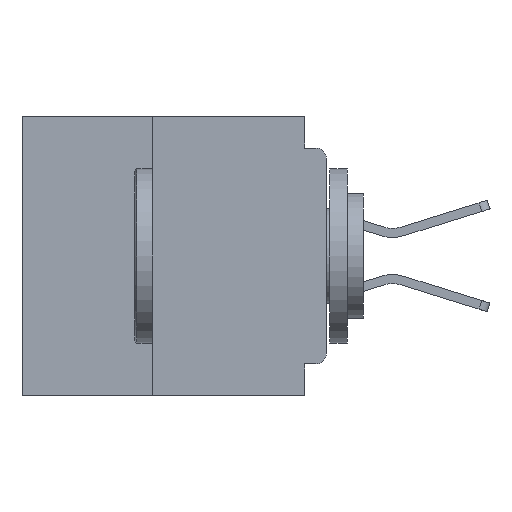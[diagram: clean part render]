
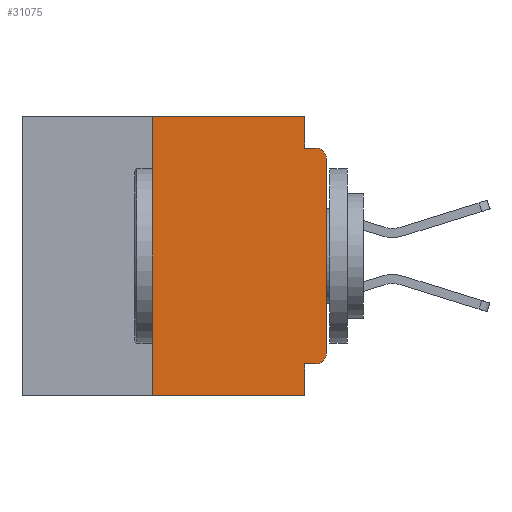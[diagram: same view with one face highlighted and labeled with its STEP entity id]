
A CAD part, left-side view. The second image highlights one B-rep face of the part: STEP entity #31075.
In plain terms, the highlighted planar face has unit normal (-1, 0, 0).
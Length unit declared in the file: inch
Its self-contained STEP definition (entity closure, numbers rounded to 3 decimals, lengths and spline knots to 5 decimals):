
#93 = CARTESIAN_POINT ( 'NONE',  ( 0., 0.015, -0.06 ) ) ;
#220 = EDGE_CURVE ( 'NONE', #1124, #21345, #11025, .T. ) ;
#912 = VERTEX_POINT ( 'NONE', #42246 ) ;
#926 = VECTOR ( 'NONE', #17626, 39.37008 ) ;
#1124 = VERTEX_POINT ( 'NONE', #22435 ) ;
#1366 = AXIS2_PLACEMENT_3D ( 'NONE', #93, #27262, #4027 ) ;
#1625 = DIRECTION ( 'NONE',  ( 0., -1., 0. ) ) ;
#2060 = ORIENTED_EDGE ( 'NONE', *, *, #20416, .F. ) ;
#3222 = CARTESIAN_POINT ( 'NONE',  ( 0., 0., -0.34 ) ) ;
#3652 = LINE ( 'NONE', #19843, #23049 ) ;
#3654 = CARTESIAN_POINT ( 'NONE',  ( 0., 0., -0.045 ) ) ;
#4017 = DIRECTION ( 'NONE',  ( 0., 0., -1. ) ) ;
#4027 = DIRECTION ( 'NONE',  ( 0., 0., -1. ) ) ;
#4839 = EDGE_CURVE ( 'NONE', #48604, #32258, #38915, .T. ) ;
#5879 = CARTESIAN_POINT ( 'NONE',  ( 0., 0.031, -0.4 ) ) ;
#5947 = CARTESIAN_POINT ( 'NONE',  ( 0., 0., -0.355 ) ) ;
#6257 = CIRCLE ( 'NONE', #8171, 0.015 ) ;
#6367 = VECTOR ( 'NONE', #1625, 39.37008 ) ;
#6814 = DIRECTION ( 'NONE',  ( 0., 0., -1. ) ) ;
#7011 = CARTESIAN_POINT ( 'NONE',  ( 0., 0.031, -0.045 ) ) ;
#7344 = EDGE_CURVE ( 'NONE', #23787, #32258, #38089, .T. ) ;
#7487 = AXIS2_PLACEMENT_3D ( 'NONE', #23342, #27258, #4017 ) ;
#8171 = AXIS2_PLACEMENT_3D ( 'NONE', #22009, #48765, #25930 ) ;
#8413 = ORIENTED_EDGE ( 'NONE', *, *, #29179, .T. ) ;
#8745 = CARTESIAN_POINT ( 'NONE',  ( 0., 0.015, -0.355 ) ) ;
#9720 = DIRECTION ( 'NONE',  ( 0., 0., 1. ) ) ;
#9764 = EDGE_CURVE ( 'NONE', #22060, #38439, #40261, .T. ) ;
#9874 = DIRECTION ( 'NONE',  ( 0., 1., 0. ) ) ;
#10141 = EDGE_CURVE ( 'NONE', #17480, #48604, #3652, .T. ) ;
#10224 = VERTEX_POINT ( 'NONE', #20346 ) ;
#11025 = LINE ( 'NONE', #42418, #12229 ) ;
#11294 = LINE ( 'NONE', #5879, #926 ) ;
#11727 = ORIENTED_EDGE ( 'NONE', *, *, #33184, .F. ) ;
#11747 = CARTESIAN_POINT ( 'NONE',  ( 0., 0.015, -0.045 ) ) ;
#12229 = VECTOR ( 'NONE', #9720, 39.37008 ) ;
#12519 = CARTESIAN_POINT ( 'NONE',  ( 0., 0.25, 0. ) ) ;
#13528 = VECTOR ( 'NONE', #6814, 39.37008 ) ;
#14479 = CARTESIAN_POINT ( 'NONE',  ( 0., 0.437, -0.4 ) ) ;
#17480 = VERTEX_POINT ( 'NONE', #3222 ) ;
#17592 = VECTOR ( 'NONE', #19287, 39.37008 ) ;
#17626 = DIRECTION ( 'NONE',  ( 0., 0., -1. ) ) ;
#18021 = ORIENTED_EDGE ( 'NONE', *, *, #9764, .F. ) ;
#18552 = ORIENTED_EDGE ( 'NONE', *, *, #23056, .F. ) ;
#19287 = DIRECTION ( 'NONE',  ( 0., -1., 0. ) ) ;
#19843 = CARTESIAN_POINT ( 'NONE',  ( 0., 0., 0. ) ) ;
#20346 = CARTESIAN_POINT ( 'NONE',  ( 0., 0.031, -0.4 ) ) ;
#20416 = EDGE_CURVE ( 'NONE', #912, #23787, #23808, .T. ) ;
#21345 = VERTEX_POINT ( 'NONE', #12519 ) ;
#22009 = CARTESIAN_POINT ( 'NONE',  ( 0., 0.015, -0.34 ) ) ;
#22060 = VERTEX_POINT ( 'NONE', #8745 ) ;
#22105 = ORIENTED_EDGE ( 'NONE', *, *, #30466, .T. ) ;
#22252 = CARTESIAN_POINT ( 'NONE',  ( 0., 0.031, 0. ) ) ;
#22435 = CARTESIAN_POINT ( 'NONE',  ( 0., 0.25, -0.4 ) ) ;
#23049 = VECTOR ( 'NONE', #23716, 39.37008 ) ;
#23056 = EDGE_CURVE ( 'NONE', #38439, #10224, #11294, .T. ) ;
#23342 = CARTESIAN_POINT ( 'NONE',  ( 0., 0.437, 0. ) ) ;
#23716 = DIRECTION ( 'NONE',  ( 0., 0., 1. ) ) ;
#23787 = VERTEX_POINT ( 'NONE', #7011 ) ;
#23808 = LINE ( 'NONE', #22252, #13528 ) ;
#23879 = CARTESIAN_POINT ( 'NONE',  ( 0., 0., -0.06 ) ) ;
#24869 = CARTESIAN_POINT ( 'NONE',  ( 0., 0.437, 0. ) ) ;
#25930 = DIRECTION ( 'NONE',  ( 0., 0., -1. ) ) ;
#27258 = DIRECTION ( 'NONE',  ( 1., 0., 0. ) ) ;
#27262 = DIRECTION ( 'NONE',  ( -1., 0., 0. ) ) ;
#28888 = VECTOR ( 'NONE', #9874, 39.37008 ) ;
#29156 = VECTOR ( 'NONE', #48982, 39.37008 ) ;
#29179 = EDGE_CURVE ( 'NONE', #22060, #17480, #6257, .T. ) ;
#30130 = ORIENTED_EDGE ( 'NONE', *, *, #10141, .T. ) ;
#30372 = LINE ( 'NONE', #14479, #29156 ) ;
#30466 = EDGE_CURVE ( 'NONE', #1124, #10224, #30372, .T. ) ;
#31075 = ADVANCED_FACE ( 'NONE', ( #41051 ), #46260, .F. ) ;
#31614 = CARTESIAN_POINT ( 'NONE',  ( 0., 0.031, -0.355 ) ) ;
#32258 = VERTEX_POINT ( 'NONE', #11747 ) ;
#32962 = ORIENTED_EDGE ( 'NONE', *, *, #220, .F. ) ;
#33184 = EDGE_CURVE ( 'NONE', #21345, #912, #46084, .T. ) ;
#37603 = ORIENTED_EDGE ( 'NONE', *, *, #7344, .F. ) ;
#38089 = LINE ( 'NONE', #3654, #17592 ) ;
#38439 = VERTEX_POINT ( 'NONE', #31614 ) ;
#38915 = CIRCLE ( 'NONE', #1366, 0.015 ) ;
#40261 = LINE ( 'NONE', #5947, #28888 ) ;
#41051 = FACE_OUTER_BOUND ( 'NONE', #47478, .T. ) ;
#42246 = CARTESIAN_POINT ( 'NONE',  ( 0., 0.031, 0. ) ) ;
#42418 = CARTESIAN_POINT ( 'NONE',  ( 0., 0.25, -0.4 ) ) ;
#46084 = LINE ( 'NONE', #24869, #6367 ) ;
#46260 = PLANE ( 'NONE',  #7487 ) ;
#47478 = EDGE_LOOP ( 'NONE', ( #30130, #48799, #37603, #2060, #11727, #32962, #22105, #18552, #18021, #8413 ) ) ;
#48604 = VERTEX_POINT ( 'NONE', #23879 ) ;
#48765 = DIRECTION ( 'NONE',  ( -1., 0., 0. ) ) ;
#48799 = ORIENTED_EDGE ( 'NONE', *, *, #4839, .T. ) ;
#48982 = DIRECTION ( 'NONE',  ( 0., -1., 0. ) ) ;
